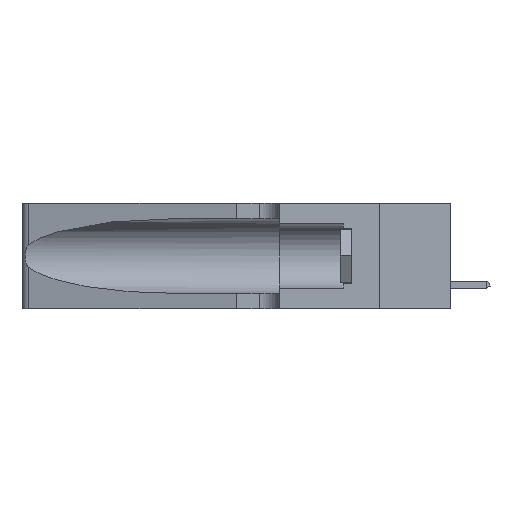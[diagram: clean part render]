
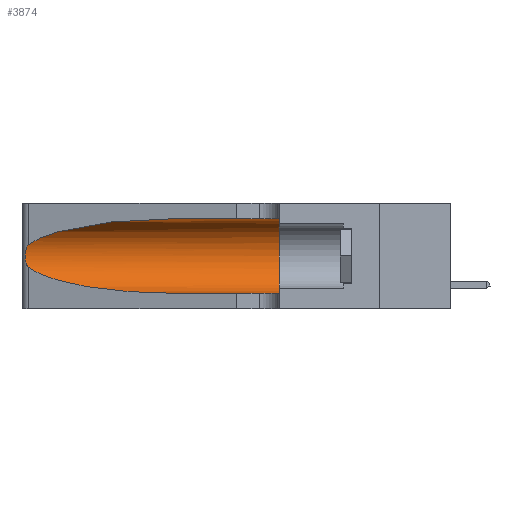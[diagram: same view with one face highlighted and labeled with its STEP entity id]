
A CAD part, left-side view. The second image highlights one B-rep face of the part: STEP entity #3874.
In plain terms, the highlighted cylindrical face has radius 3.308 mm (diameter 6.617 mm), a partial arc.
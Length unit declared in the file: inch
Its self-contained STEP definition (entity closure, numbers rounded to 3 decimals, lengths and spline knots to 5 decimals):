
#654 = DIRECTION ( 'NONE',  ( 0., 0., 1. ) ) ;
#858 = CARTESIAN_POINT ( 'NONE',  ( 0.1305, 0.35, 0.31525 ) ) ;
#1111 = ORIENTED_EDGE ( 'NONE', *, *, #25598, .T. ) ;
#1868 = CARTESIAN_POINT ( 'NONE',  ( 0.26018, 1.23835, 0.19895 ) ) ;
#2016 = VERTEX_POINT ( 'NONE', #20028 ) ;
#3487 = FACE_OUTER_BOUND ( 'NONE', #36163, .T. ) ;
#3733 = CARTESIAN_POINT ( 'NONE',  ( 0.25487, 1.22718, 0.22369 ) ) ;
#3874 = ADVANCED_FACE ( 'NONE', ( #3487 ), #45399, .F. ) ;
#4853 = VERTEX_POINT ( 'NONE', #16607 ) ;
#7282 = EDGE_CURVE ( 'NONE', #4853, #2016, #13872, .T. ) ;
#7424 =( BOUNDED_CURVE ( )  B_SPLINE_CURVE ( 3, ( #40626, #30207, #8477, #34208 ),
 .UNSPECIFIED., .F., .F. ) 
 B_SPLINE_CURVE_WITH_KNOTS ( ( 4, 4 ),
 ( 1.5708, 2.84003 ),
 .UNSPECIFIED. ) 
 CURVE ( )  GEOMETRIC_REPRESENTATION_ITEM ( )  RATIONAL_B_SPLINE_CURVE ( ( 1., 0.87, 0.87, 1. ) ) 
 REPRESENTATION_ITEM ( '' )  );
#7536 = CARTESIAN_POINT ( 'NONE',  ( 0.26075, 1.23896, 0.178 ) ) ;
#8303 = VECTOR ( 'NONE', #46304, 39.37008 ) ;
#8477 = CARTESIAN_POINT ( 'NONE',  ( 0.2373, 1.15595, 0.28018 ) ) ;
#8517 = AXIS2_PLACEMENT_3D ( 'NONE', #21018, #32141, #654 ) ;
#8986 = EDGE_CURVE ( 'NONE', #45056, #4853, #10382, .T. ) ;
#9091 = CARTESIAN_POINT ( 'NONE',  ( 0.25787, 1.23484, 0.2124 ) ) ;
#10047 = CARTESIAN_POINT ( 'NONE',  ( 0.25854, 1.2359, 0.20912 ) ) ;
#10082 = CARTESIAN_POINT ( 'NONE',  ( 0.26075, 1.23896, 0.19203 ) ) ;
#10332 = CIRCLE ( 'NONE', #8517, 0.13025 ) ;
#10381 = VECTOR ( 'NONE', #40699, 39.37008 ) ;
#10382 = B_SPLINE_CURVE_WITH_KNOTS ( 'NONE', 3,
 ( #39666, #16055, #19714, #9091, #10047, #1868, #10082, #7536, #45381, #19484, #34486, #35259, #45057, #33730 ),
 .UNSPECIFIED., .F., .F.,
 ( 4, 2, 2, 2, 2, 2, 4 ),
 ( 0., 0.00027, 0.00053, 0.00107, 0.0016, 0.00187, 0.00214 ),
 .UNSPECIFIED. ) ;
#12551 = ORIENTED_EDGE ( 'NONE', *, *, #8986, .T. ) ;
#12610 = LINE ( 'NONE', #25951, #10381 ) ;
#13872 =( BOUNDED_CURVE ( )  B_SPLINE_CURVE ( 3, ( #38235, #20192, #16707, #27624 ),
 .UNSPECIFIED., .F., .T. ) 
 B_SPLINE_CURVE_WITH_KNOTS ( ( 4, 4 ),
 ( 3.44316, 4.71239 ),
 .UNSPECIFIED. ) 
 CURVE ( )  GEOMETRIC_REPRESENTATION_ITEM ( )  RATIONAL_B_SPLINE_CURVE ( ( 1., 0.87, 0.87, 1. ) ) 
 REPRESENTATION_ITEM ( '' )  );
#14012 = AXIS2_PLACEMENT_3D ( 'NONE', #24761, #14133, #39754 ) ;
#14133 = DIRECTION ( 'NONE',  ( 0., -1., 0. ) ) ;
#15292 = EDGE_CURVE ( 'NONE', #26472, #45056, #7424, .T. ) ;
#16055 = CARTESIAN_POINT ( 'NONE',  ( 0.25555, 1.22994, 0.2215 ) ) ;
#16607 = CARTESIAN_POINT ( 'NONE',  ( 0.25487, 1.22718, 0.14631 ) ) ;
#16707 = CARTESIAN_POINT ( 'NONE',  ( 0.18966, 0.96281, 0.05475 ) ) ;
#18333 = CARTESIAN_POINT ( 'NONE',  ( 0.1305, 1.61858, 0.31525 ) ) ;
#18912 = EDGE_CURVE ( 'NONE', #26472, #25669, #23090, .T. ) ;
#19484 = CARTESIAN_POINT ( 'NONE',  ( 0.25856, 1.23593, 0.16098 ) ) ;
#19714 = CARTESIAN_POINT ( 'NONE',  ( 0.25639, 1.23184, 0.21858 ) ) ;
#20028 = CARTESIAN_POINT ( 'NONE',  ( 0.1305, 0.72297, 0.05475 ) ) ;
#20192 = CARTESIAN_POINT ( 'NONE',  ( 0.2373, 1.15595, 0.08982 ) ) ;
#21009 = ORIENTED_EDGE ( 'NONE', *, *, #26025, .F. ) ;
#21018 = CARTESIAN_POINT ( 'NONE',  ( 0.1305, 0.35, 0.185 ) ) ;
#22344 = ORIENTED_EDGE ( 'NONE', *, *, #7282, .T. ) ;
#22856 = VERTEX_POINT ( 'NONE', #37192 ) ;
#23090 = LINE ( 'NONE', #18333, #8303 ) ;
#24761 = CARTESIAN_POINT ( 'NONE',  ( 0.1305, 1.61858, 0.185 ) ) ;
#25598 = EDGE_CURVE ( 'NONE', #2016, #22856, #12610, .T. ) ;
#25669 = VERTEX_POINT ( 'NONE', #858 ) ;
#25951 = CARTESIAN_POINT ( 'NONE',  ( 0.1305, 1.61858, 0.05475 ) ) ;
#26025 = EDGE_CURVE ( 'NONE', #25669, #22856, #10332, .T. ) ;
#26260 = ORIENTED_EDGE ( 'NONE', *, *, #18912, .F. ) ;
#26472 = VERTEX_POINT ( 'NONE', #31204 ) ;
#27624 = CARTESIAN_POINT ( 'NONE',  ( 0.1305, 0.72297, 0.05475 ) ) ;
#30145 = ORIENTED_EDGE ( 'NONE', *, *, #15292, .T. ) ;
#30207 = CARTESIAN_POINT ( 'NONE',  ( 0.18966, 0.96281, 0.31525 ) ) ;
#31204 = CARTESIAN_POINT ( 'NONE',  ( 0.1305, 0.72297, 0.31525 ) ) ;
#32141 = DIRECTION ( 'NONE',  ( 0., 1., 0. ) ) ;
#33730 = CARTESIAN_POINT ( 'NONE',  ( 0.25487, 1.22718, 0.14631 ) ) ;
#34208 = CARTESIAN_POINT ( 'NONE',  ( 0.25487, 1.22718, 0.22369 ) ) ;
#34486 = CARTESIAN_POINT ( 'NONE',  ( 0.25789, 1.23486, 0.15765 ) ) ;
#35259 = CARTESIAN_POINT ( 'NONE',  ( 0.25639, 1.23186, 0.15144 ) ) ;
#36163 = EDGE_LOOP ( 'NONE', ( #30145, #12551, #22344, #1111, #21009, #26260 ) ) ;
#37192 = CARTESIAN_POINT ( 'NONE',  ( 0.1305, 0.35, 0.05475 ) ) ;
#38235 = CARTESIAN_POINT ( 'NONE',  ( 0.25487, 1.22718, 0.14631 ) ) ;
#39666 = CARTESIAN_POINT ( 'NONE',  ( 0.25487, 1.22718, 0.22369 ) ) ;
#39754 = DIRECTION ( 'NONE',  ( 0., 0., -1. ) ) ;
#40626 = CARTESIAN_POINT ( 'NONE',  ( 0.1305, 0.72297, 0.31525 ) ) ;
#40699 = DIRECTION ( 'NONE',  ( 0., -1., 0. ) ) ;
#45056 = VERTEX_POINT ( 'NONE', #3733 ) ;
#45057 = CARTESIAN_POINT ( 'NONE',  ( 0.25555, 1.22993, 0.14849 ) ) ;
#45381 = CARTESIAN_POINT ( 'NONE',  ( 0.26017, 1.23833, 0.17102 ) ) ;
#45399 = CYLINDRICAL_SURFACE ( 'NONE', #14012, 0.13025 ) ;
#46304 = DIRECTION ( 'NONE',  ( 0., -1., 0. ) ) ;
